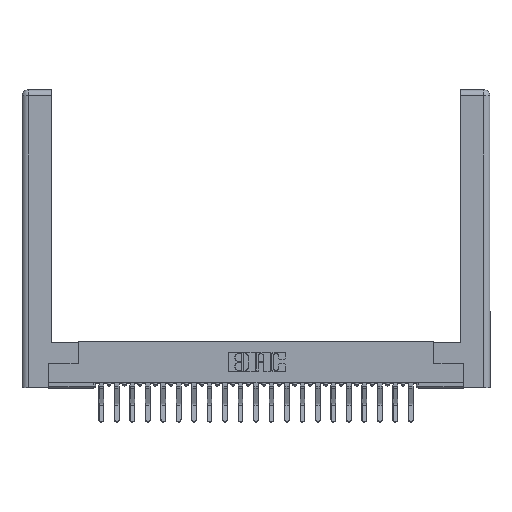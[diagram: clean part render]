
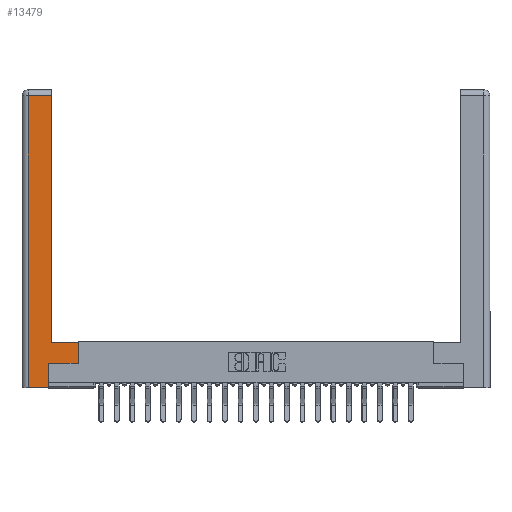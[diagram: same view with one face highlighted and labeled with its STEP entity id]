
A CAD part, top view. The second image highlights one B-rep face of the part: STEP entity #13479.
In plain terms, the highlighted planar face has unit normal (0, 0, 1).
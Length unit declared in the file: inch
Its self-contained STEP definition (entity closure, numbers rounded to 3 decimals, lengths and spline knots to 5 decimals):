
#555 = LINE ( 'NONE', #6510, #21201 ) ;
#1482 = VERTEX_POINT ( 'NONE', #22295 ) ;
#1546 = EDGE_CURVE ( 'NONE', #16616, #15737, #555, .T. ) ;
#1567 = LINE ( 'NONE', #3378, #5952 ) ;
#1669 = LINE ( 'NONE', #18174, #22300 ) ;
#2852 = VERTEX_POINT ( 'NONE', #9837 ) ;
#2958 = CARTESIAN_POINT ( 'NONE',  ( 0.565, 0.45, 0. ) ) ;
#2992 = VERTEX_POINT ( 'NONE', #8718 ) ;
#3028 = VERTEX_POINT ( 'NONE', #19642 ) ;
#3176 = CARTESIAN_POINT ( 'NONE',  ( 0.0615, 2.94, 0. ) ) ;
#3366 = ORIENTED_EDGE ( 'NONE', *, *, #18726, .T. ) ;
#3378 = CARTESIAN_POINT ( 'NONE',  ( 0.295, 3., 0. ) ) ;
#3406 = ORIENTED_EDGE ( 'NONE', *, *, #22026, .T. ) ;
#3431 = EDGE_CURVE ( 'NONE', #2852, #16616, #10468, .T. ) ;
#5952 = VECTOR ( 'NONE', #14200, 39.37008 ) ;
#6081 = VERTEX_POINT ( 'NONE', #22601 ) ;
#6510 = CARTESIAN_POINT ( 'NONE',  ( 0.0615, 0., 0. ) ) ;
#7004 = EDGE_LOOP ( 'NONE', ( #3406, #15454, #23423, #14214, #21990, #22184, #8735, #3366 ) ) ;
#7972 = DIRECTION ( 'NONE',  ( 0., -1., 0. ) ) ;
#8377 = LINE ( 'NONE', #23168, #18551 ) ;
#8718 = CARTESIAN_POINT ( 'NONE',  ( 0.295, 0.45, 0. ) ) ;
#8735 = ORIENTED_EDGE ( 'NONE', *, *, #13465, .T. ) ;
#9211 = CARTESIAN_POINT ( 'NONE',  ( 0.265, 0., 0. ) ) ;
#9339 = EDGE_CURVE ( 'NONE', #15737, #6081, #21704, .T. ) ;
#9837 = CARTESIAN_POINT ( 'NONE',  ( 0.295, 2.94, 0. ) ) ;
#10468 = LINE ( 'NONE', #3176, #11731 ) ;
#10621 = CARTESIAN_POINT ( 'NONE',  ( 0.565, 0.245, 0. ) ) ;
#11029 = DIRECTION ( 'NONE',  ( 0., 1., 0. ) ) ;
#11614 = CARTESIAN_POINT ( 'NONE',  ( 0.0615, 0., 0. ) ) ;
#11689 = VECTOR ( 'NONE', #16085, 39.37008 ) ;
#11731 = VECTOR ( 'NONE', #17758, 39.37008 ) ;
#11839 = LINE ( 'NONE', #2958, #11689 ) ;
#12779 = LINE ( 'NONE', #20207, #21730 ) ;
#13465 = EDGE_CURVE ( 'NONE', #13714, #1482, #11839, .T. ) ;
#13479 = ADVANCED_FACE ( 'NONE', ( #15732 ), #21303, .F. ) ;
#13714 = VERTEX_POINT ( 'NONE', #10621 ) ;
#13926 = DIRECTION ( 'NONE',  ( 1., 0., 0. ) ) ;
#14200 = DIRECTION ( 'NONE',  ( 0., 1., 0. ) ) ;
#14214 = ORIENTED_EDGE ( 'NONE', *, *, #9339, .T. ) ;
#14683 = VECTOR ( 'NONE', #24016, 39.37008 ) ;
#15454 = ORIENTED_EDGE ( 'NONE', *, *, #3431, .T. ) ;
#15474 = EDGE_CURVE ( 'NONE', #3028, #13714, #8377, .T. ) ;
#15732 = FACE_OUTER_BOUND ( 'NONE', #7004, .T. ) ;
#15737 = VERTEX_POINT ( 'NONE', #11614 ) ;
#16085 = DIRECTION ( 'NONE',  ( 0., 1., 0. ) ) ;
#16616 = VERTEX_POINT ( 'NONE', #17481 ) ;
#17481 = CARTESIAN_POINT ( 'NONE',  ( 0.0615, 2.94, 0. ) ) ;
#17758 = DIRECTION ( 'NONE',  ( -1., 0., 0. ) ) ;
#18174 = CARTESIAN_POINT ( 'NONE',  ( 0.265, 0.245, 0. ) ) ;
#18551 = VECTOR ( 'NONE', #13926, 39.37008 ) ;
#18726 = EDGE_CURVE ( 'NONE', #1482, #2992, #12779, .T. ) ;
#19258 = DIRECTION ( 'NONE',  ( 0., 0., -1. ) ) ;
#19365 = DIRECTION ( 'NONE',  ( -1., 0., 0. ) ) ;
#19455 = AXIS2_PLACEMENT_3D ( 'NONE', #23372, #19258, #19365 ) ;
#19642 = CARTESIAN_POINT ( 'NONE',  ( 0.265, 0.245, 0. ) ) ;
#20207 = CARTESIAN_POINT ( 'NONE',  ( 0.295, 0.45, 0. ) ) ;
#21201 = VECTOR ( 'NONE', #7972, 39.37008 ) ;
#21303 = PLANE ( 'NONE',  #19455 ) ;
#21704 = LINE ( 'NONE', #9211, #14683 ) ;
#21730 = VECTOR ( 'NONE', #22270, 39.37008 ) ;
#21990 = ORIENTED_EDGE ( 'NONE', *, *, #23811, .T. ) ;
#22026 = EDGE_CURVE ( 'NONE', #2992, #2852, #1567, .T. ) ;
#22184 = ORIENTED_EDGE ( 'NONE', *, *, #15474, .T. ) ;
#22270 = DIRECTION ( 'NONE',  ( -1., 0., 0. ) ) ;
#22295 = CARTESIAN_POINT ( 'NONE',  ( 0.565, 0.45, 0. ) ) ;
#22300 = VECTOR ( 'NONE', #11029, 39.37008 ) ;
#22601 = CARTESIAN_POINT ( 'NONE',  ( 0.265, 0., 0. ) ) ;
#23168 = CARTESIAN_POINT ( 'NONE',  ( 0.565, 0.245, 0. ) ) ;
#23372 = CARTESIAN_POINT ( 'NONE',  ( 0., 0., 0. ) ) ;
#23423 = ORIENTED_EDGE ( 'NONE', *, *, #1546, .T. ) ;
#23811 = EDGE_CURVE ( 'NONE', #6081, #3028, #1669, .T. ) ;
#24016 = DIRECTION ( 'NONE',  ( 1., 0., 0. ) ) ;
